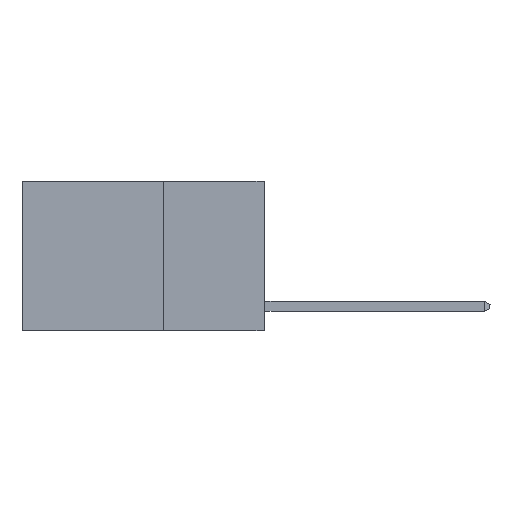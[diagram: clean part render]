
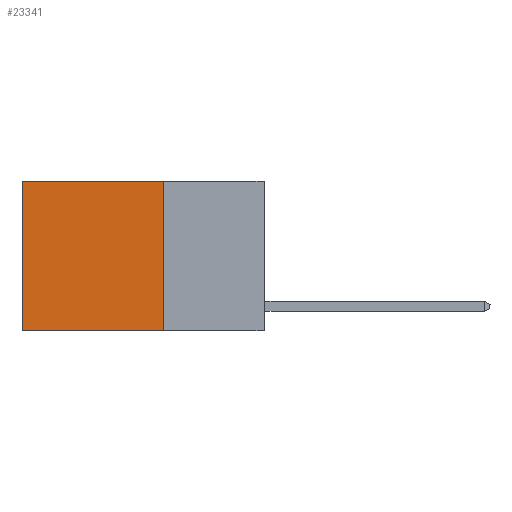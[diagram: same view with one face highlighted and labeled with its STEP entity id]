
A CAD part, left-side view. The second image highlights one B-rep face of the part: STEP entity #23341.
In plain terms, the highlighted planar face has unit normal (-1, 0, 0).
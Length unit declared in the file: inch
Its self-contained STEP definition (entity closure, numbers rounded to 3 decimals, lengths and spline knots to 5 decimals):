
#2438 = CARTESIAN_POINT ( 'NONE',  ( 0.2625, 0.25, 0. ) ) ;
#2613 = VECTOR ( 'NONE', #19914, 39.37008 ) ;
#2910 = VECTOR ( 'NONE', #18129, 39.37008 ) ;
#3908 = EDGE_CURVE ( 'NONE', #6506, #8686, #17496, .T. ) ;
#5279 = ORIENTED_EDGE ( 'NONE', *, *, #5442, .F. ) ;
#5442 = EDGE_CURVE ( 'NONE', #8686, #7321, #16487, .T. ) ;
#6104 = LINE ( 'NONE', #6697, #20276 ) ;
#6506 = VERTEX_POINT ( 'NONE', #19430 ) ;
#6697 = CARTESIAN_POINT ( 'NONE',  ( 0.2625, 0.25, 0. ) ) ;
#6969 = CARTESIAN_POINT ( 'NONE',  ( 0.2625, 0.6, -0.37 ) ) ;
#7321 = VERTEX_POINT ( 'NONE', #6969 ) ;
#8686 = VERTEX_POINT ( 'NONE', #11430 ) ;
#9433 = ORIENTED_EDGE ( 'NONE', *, *, #3908, .F. ) ;
#10840 = VECTOR ( 'NONE', #16668, 39.37008 ) ;
#10907 = DIRECTION ( 'NONE',  ( 0., 1., 0. ) ) ;
#11430 = CARTESIAN_POINT ( 'NONE',  ( 0.2625, 0.25, -0.37 ) ) ;
#12004 = EDGE_LOOP ( 'NONE', ( #14057, #5279, #9433, #24556 ) ) ;
#13078 = DIRECTION ( 'NONE',  ( 0., 0., -1. ) ) ;
#14057 = ORIENTED_EDGE ( 'NONE', *, *, #16727, .T. ) ;
#16487 = LINE ( 'NONE', #20373, #2910 ) ;
#16668 = DIRECTION ( 'NONE',  ( 0., 0., -1. ) ) ;
#16727 = EDGE_CURVE ( 'NONE', #25567, #7321, #20278, .T. ) ;
#17496 = LINE ( 'NONE', #2438, #10840 ) ;
#17836 = CARTESIAN_POINT ( 'NONE',  ( 0.2625, 0.6, 0. ) ) ;
#18129 = DIRECTION ( 'NONE',  ( 0., 1., 0. ) ) ;
#19430 = CARTESIAN_POINT ( 'NONE',  ( 0.2625, 0.25, 0. ) ) ;
#19755 = FACE_OUTER_BOUND ( 'NONE', #12004, .T. ) ;
#19914 = DIRECTION ( 'NONE',  ( 0., 0., -1. ) ) ;
#20056 = EDGE_CURVE ( 'NONE', #6506, #25567, #6104, .T. ) ;
#20276 = VECTOR ( 'NONE', #10907, 39.37008 ) ;
#20278 = LINE ( 'NONE', #17836, #2613 ) ;
#20373 = CARTESIAN_POINT ( 'NONE',  ( 0.2625, 0.25, -0.37 ) ) ;
#20973 = CARTESIAN_POINT ( 'NONE',  ( 0.2625, 0.25, 0. ) ) ;
#21692 = CARTESIAN_POINT ( 'NONE',  ( 0.2625, 0.6, 0. ) ) ;
#22319 = AXIS2_PLACEMENT_3D ( 'NONE', #20973, #25018, #13078 ) ;
#23341 = ADVANCED_FACE ( 'NONE', ( #19755 ), #24758, .F. ) ;
#24556 = ORIENTED_EDGE ( 'NONE', *, *, #20056, .T. ) ;
#24758 = PLANE ( 'NONE',  #22319 ) ;
#25018 = DIRECTION ( 'NONE',  ( 1., 0., 0. ) ) ;
#25567 = VERTEX_POINT ( 'NONE', #21692 ) ;
